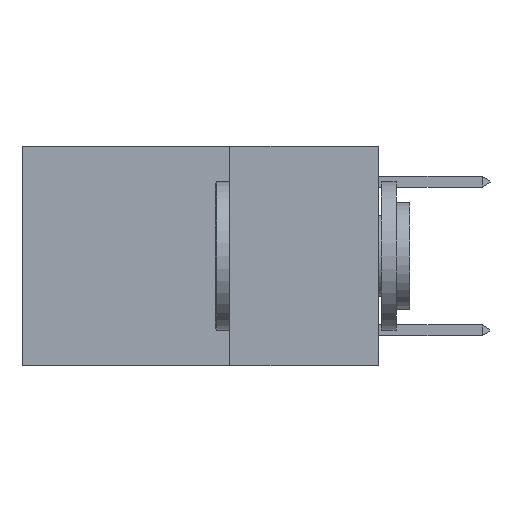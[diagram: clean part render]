
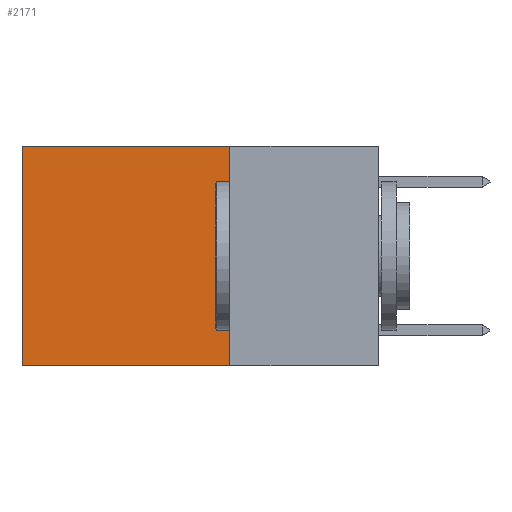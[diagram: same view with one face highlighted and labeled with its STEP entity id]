
A CAD part, left-side view. The second image highlights one B-rep face of the part: STEP entity #2171.
In plain terms, the highlighted planar face has unit normal (-1, 0, 0).
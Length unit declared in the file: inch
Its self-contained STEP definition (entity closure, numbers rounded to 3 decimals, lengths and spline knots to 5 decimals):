
#761 = VECTOR ( 'NONE', #12226, 39.37008 ) ;
#770 = VECTOR ( 'NONE', #9620, 39.37008 ) ;
#1097 = VECTOR ( 'NONE', #16054, 39.37008 ) ;
#1279 = EDGE_CURVE ( 'NONE', #9114, #15926, #6427, .T. ) ;
#1434 = ORIENTED_EDGE ( 'NONE', *, *, #4837, .F. ) ;
#1797 = EDGE_CURVE ( 'NONE', #9114, #2885, #11948, .T. ) ;
#2171 = ADVANCED_FACE ( 'NONE', ( #12160 ), #14571, .F. ) ;
#2382 = VECTOR ( 'NONE', #5103, 39.37008 ) ;
#2688 = ORIENTED_EDGE ( 'NONE', *, *, #1279, .T. ) ;
#2885 = VERTEX_POINT ( 'NONE', #12108 ) ;
#3847 = CARTESIAN_POINT ( 'NONE',  ( 0.2625, 0.25, 0. ) ) ;
#4643 = CARTESIAN_POINT ( 'NONE',  ( 0.2625, 0.25, 0. ) ) ;
#4837 = EDGE_CURVE ( 'NONE', #2885, #5179, #7577, .T. ) ;
#5103 = DIRECTION ( 'NONE',  ( 0., 1., 0. ) ) ;
#5179 = VERTEX_POINT ( 'NONE', #12151 ) ;
#5186 = CARTESIAN_POINT ( 'NONE',  ( 0.2625, 0.25, -0.37 ) ) ;
#5659 = EDGE_LOOP ( 'NONE', ( #8251, #1434, #6215, #2688 ) ) ;
#6061 = CARTESIAN_POINT ( 'NONE',  ( 0.2625, 0.6, 0. ) ) ;
#6215 = ORIENTED_EDGE ( 'NONE', *, *, #1797, .F. ) ;
#6427 = LINE ( 'NONE', #12564, #2382 ) ;
#7399 = DIRECTION ( 'NONE',  ( 1., 0., 0. ) ) ;
#7577 = LINE ( 'NONE', #5186, #1097 ) ;
#8251 = ORIENTED_EDGE ( 'NONE', *, *, #13248, .T. ) ;
#8446 = CARTESIAN_POINT ( 'NONE',  ( 0.2625, 0.25, 0. ) ) ;
#9114 = VERTEX_POINT ( 'NONE', #4643 ) ;
#9620 = DIRECTION ( 'NONE',  ( 0., 0., -1. ) ) ;
#9823 = DIRECTION ( 'NONE',  ( 0., 0., -1. ) ) ;
#11227 = CARTESIAN_POINT ( 'NONE',  ( 0.2625, 0.6, 0. ) ) ;
#11948 = LINE ( 'NONE', #8446, #770 ) ;
#12108 = CARTESIAN_POINT ( 'NONE',  ( 0.2625, 0.25, -0.37 ) ) ;
#12151 = CARTESIAN_POINT ( 'NONE',  ( 0.2625, 0.6, -0.37 ) ) ;
#12160 = FACE_OUTER_BOUND ( 'NONE', #5659, .T. ) ;
#12226 = DIRECTION ( 'NONE',  ( 0., 0., -1. ) ) ;
#12564 = CARTESIAN_POINT ( 'NONE',  ( 0.2625, 0.25, 0. ) ) ;
#13248 = EDGE_CURVE ( 'NONE', #15926, #5179, #13497, .T. ) ;
#13497 = LINE ( 'NONE', #11227, #761 ) ;
#14383 = AXIS2_PLACEMENT_3D ( 'NONE', #3847, #7399, #9823 ) ;
#14571 = PLANE ( 'NONE',  #14383 ) ;
#15926 = VERTEX_POINT ( 'NONE', #6061 ) ;
#16054 = DIRECTION ( 'NONE',  ( 0., 1., 0. ) ) ;
